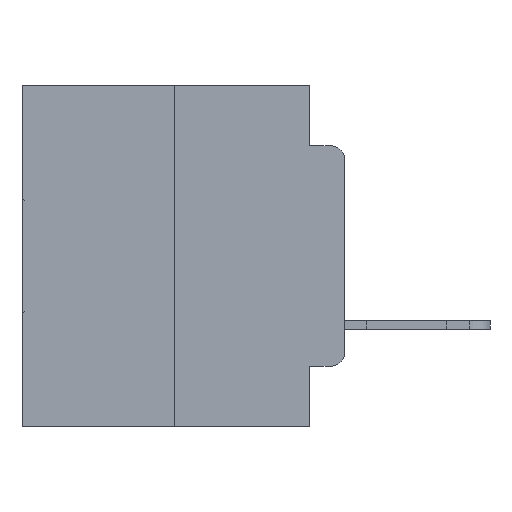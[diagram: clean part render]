
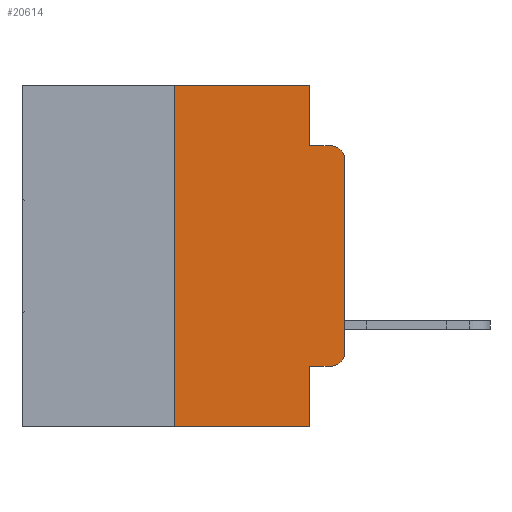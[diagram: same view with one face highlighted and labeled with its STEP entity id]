
A CAD part, left-side view. The second image highlights one B-rep face of the part: STEP entity #20614.
In plain terms, the highlighted planar face has unit normal (-1, 0, 0).
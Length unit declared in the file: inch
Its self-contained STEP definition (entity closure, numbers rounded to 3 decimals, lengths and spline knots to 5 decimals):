
#132 = EDGE_CURVE ( 'NONE', #28459, #23200, #11867, .T. ) ;
#237 = ORIENTED_EDGE ( 'NONE', *, *, #10905, .F. ) ;
#588 = DIRECTION ( 'NONE',  ( 0., 0., 1. ) ) ;
#1231 = CARTESIAN_POINT ( 'NONE',  ( 0., 0.02, -0.4115 ) ) ;
#2021 = ORIENTED_EDGE ( 'NONE', *, *, #13554, .T. ) ;
#2071 = VERTEX_POINT ( 'NONE', #2554 ) ;
#2554 = CARTESIAN_POINT ( 'NONE',  ( 0., 0.25, 0. ) ) ;
#2772 = VERTEX_POINT ( 'NONE', #4872 ) ;
#2838 = DIRECTION ( 'NONE',  ( 0., -1., 0. ) ) ;
#2849 = VERTEX_POINT ( 'NONE', #7605 ) ;
#3168 = VECTOR ( 'NONE', #2838, 39.37008 ) ;
#3273 = EDGE_CURVE ( 'NONE', #2849, #29588, #17522, .T. ) ;
#3642 = CIRCLE ( 'NONE', #3680, 0.02 ) ;
#3656 = CARTESIAN_POINT ( 'NONE',  ( 0., 0.25, -0.5 ) ) ;
#3680 = AXIS2_PLACEMENT_3D ( 'NONE', #17341, #24284, #10482 ) ;
#4605 = PLANE ( 'NONE',  #12182 ) ;
#4754 = LINE ( 'NONE', #14995, #18084 ) ;
#4872 = CARTESIAN_POINT ( 'NONE',  ( 0., 0.02, -0.0885 ) ) ;
#4960 = LINE ( 'NONE', #28102, #3168 ) ;
#5169 = VERTEX_POINT ( 'NONE', #8289 ) ;
#6236 = ORIENTED_EDGE ( 'NONE', *, *, #12324, .F. ) ;
#7111 = CARTESIAN_POINT ( 'NONE',  ( 0., 0.051, -0.5 ) ) ;
#7275 = CARTESIAN_POINT ( 'NONE',  ( 0., 0.051, -0.0885 ) ) ;
#7605 = CARTESIAN_POINT ( 'NONE',  ( 0., 0.051, 0. ) ) ;
#8289 = CARTESIAN_POINT ( 'NONE',  ( 0., 0., -0.1085 ) ) ;
#8461 = EDGE_CURVE ( 'NONE', #29588, #2772, #4960, .T. ) ;
#8480 = EDGE_CURVE ( 'NONE', #5169, #2772, #11085, .T. ) ;
#9449 = DIRECTION ( 'NONE',  ( 0., -1., 0. ) ) ;
#9988 = CARTESIAN_POINT ( 'NONE',  ( 0., 0., 0. ) ) ;
#10482 = DIRECTION ( 'NONE',  ( 0., 0., -1. ) ) ;
#10602 = CARTESIAN_POINT ( 'NONE',  ( 0., 0.051, -0.4115 ) ) ;
#10605 = VERTEX_POINT ( 'NONE', #15738 ) ;
#10905 = EDGE_CURVE ( 'NONE', #2071, #2849, #26606, .T. ) ;
#11085 = CIRCLE ( 'NONE', #14504, 0.02 ) ;
#11375 = DIRECTION ( 'NONE',  ( 0., 0., -1. ) ) ;
#11440 = CARTESIAN_POINT ( 'NONE',  ( 0., 0.473, -0.5 ) ) ;
#11867 = LINE ( 'NONE', #11440, #23391 ) ;
#12182 = AXIS2_PLACEMENT_3D ( 'NONE', #14029, #16368, #20797 ) ;
#12207 = VERTEX_POINT ( 'NONE', #18950 ) ;
#12324 = EDGE_CURVE ( 'NONE', #28459, #2071, #4754, .T. ) ;
#12383 = ORIENTED_EDGE ( 'NONE', *, *, #25973, .T. ) ;
#12552 = VECTOR ( 'NONE', #15282, 39.37008 ) ;
#13383 = CARTESIAN_POINT ( 'NONE',  ( 0., 0.051, 0. ) ) ;
#13554 = EDGE_CURVE ( 'NONE', #12207, #23447, #27347, .T. ) ;
#13972 = ORIENTED_EDGE ( 'NONE', *, *, #25878, .F. ) ;
#14029 = CARTESIAN_POINT ( 'NONE',  ( 0., 0.473, 0. ) ) ;
#14170 = DIRECTION ( 'NONE',  ( 0., 0., -1. ) ) ;
#14504 = AXIS2_PLACEMENT_3D ( 'NONE', #26714, #26819, #22279 ) ;
#14995 = CARTESIAN_POINT ( 'NONE',  ( 0., 0.25, 0. ) ) ;
#15034 = ORIENTED_EDGE ( 'NONE', *, *, #8461, .F. ) ;
#15251 = VECTOR ( 'NONE', #27139, 39.37008 ) ;
#15282 = DIRECTION ( 'NONE',  ( 0., -1., 0. ) ) ;
#15738 = CARTESIAN_POINT ( 'NONE',  ( 0., 0., -0.3915 ) ) ;
#16055 = VECTOR ( 'NONE', #11375, 39.37008 ) ;
#16368 = DIRECTION ( 'NONE',  ( 1., 0., 0. ) ) ;
#17341 = CARTESIAN_POINT ( 'NONE',  ( 0., 0.02, -0.3915 ) ) ;
#17522 = LINE ( 'NONE', #13383, #16055 ) ;
#17671 = CARTESIAN_POINT ( 'NONE',  ( 0., 0.473, 0. ) ) ;
#18084 = VECTOR ( 'NONE', #19559, 39.37008 ) ;
#18723 = VECTOR ( 'NONE', #14170, 39.37008 ) ;
#18840 = LINE ( 'NONE', #9988, #25690 ) ;
#18950 = CARTESIAN_POINT ( 'NONE',  ( 0., 0.051, -0.4115 ) ) ;
#19559 = DIRECTION ( 'NONE',  ( 0., 0., 1. ) ) ;
#19694 = EDGE_CURVE ( 'NONE', #10605, #5169, #18840, .T. ) ;
#20002 = ORIENTED_EDGE ( 'NONE', *, *, #3273, .F. ) ;
#20559 = LINE ( 'NONE', #21133, #18723 ) ;
#20614 = ADVANCED_FACE ( 'NONE', ( #20975 ), #4605, .F. ) ;
#20797 = DIRECTION ( 'NONE',  ( 0., 0., -1. ) ) ;
#20975 = FACE_OUTER_BOUND ( 'NONE', #29733, .T. ) ;
#21133 = CARTESIAN_POINT ( 'NONE',  ( 0., 0.051, 0. ) ) ;
#22279 = DIRECTION ( 'NONE',  ( 0., 0., -1. ) ) ;
#23097 = ORIENTED_EDGE ( 'NONE', *, *, #132, .T. ) ;
#23200 = VERTEX_POINT ( 'NONE', #7111 ) ;
#23391 = VECTOR ( 'NONE', #9449, 39.37008 ) ;
#23447 = VERTEX_POINT ( 'NONE', #1231 ) ;
#24284 = DIRECTION ( 'NONE',  ( -1., 0., 0. ) ) ;
#25690 = VECTOR ( 'NONE', #588, 39.37008 ) ;
#25878 = EDGE_CURVE ( 'NONE', #12207, #23200, #20559, .T. ) ;
#25973 = EDGE_CURVE ( 'NONE', #23447, #10605, #3642, .T. ) ;
#26606 = LINE ( 'NONE', #17671, #15251 ) ;
#26714 = CARTESIAN_POINT ( 'NONE',  ( 0., 0.02, -0.1085 ) ) ;
#26819 = DIRECTION ( 'NONE',  ( -1., 0., 0. ) ) ;
#26973 = ORIENTED_EDGE ( 'NONE', *, *, #8480, .T. ) ;
#27139 = DIRECTION ( 'NONE',  ( 0., -1., 0. ) ) ;
#27347 = LINE ( 'NONE', #10602, #12552 ) ;
#28102 = CARTESIAN_POINT ( 'NONE',  ( 0., 0.051, -0.0885 ) ) ;
#28459 = VERTEX_POINT ( 'NONE', #3656 ) ;
#29494 = ORIENTED_EDGE ( 'NONE', *, *, #19694, .T. ) ;
#29588 = VERTEX_POINT ( 'NONE', #7275 ) ;
#29733 = EDGE_LOOP ( 'NONE', ( #29494, #26973, #15034, #20002, #237, #6236, #23097, #13972, #2021, #12383 ) ) ;
